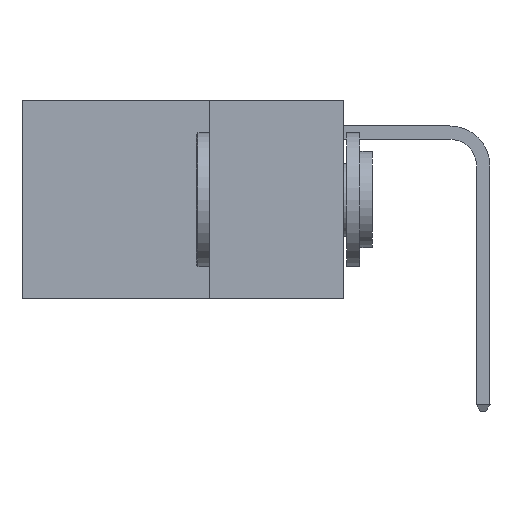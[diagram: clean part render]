
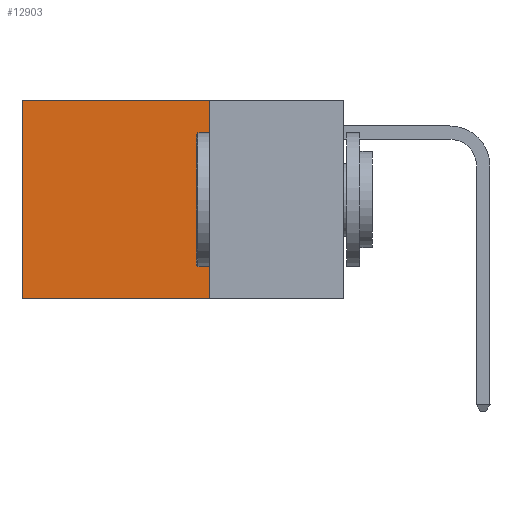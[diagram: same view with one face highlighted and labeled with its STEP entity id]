
A CAD part, left-side view. The second image highlights one B-rep face of the part: STEP entity #12903.
In plain terms, the highlighted planar face has unit normal (-1, 0, 0).
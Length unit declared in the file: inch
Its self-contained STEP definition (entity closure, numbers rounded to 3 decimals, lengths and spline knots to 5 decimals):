
#828 = CARTESIAN_POINT ( 'NONE',  ( 0.2625, 0.25, -0.37 ) ) ;
#1085 = VECTOR ( 'NONE', #15985, 39.37008 ) ;
#1234 = LINE ( 'NONE', #3697, #1085 ) ;
#2043 = ORIENTED_EDGE ( 'NONE', *, *, #5009, .T. ) ;
#2195 = ORIENTED_EDGE ( 'NONE', *, *, #12902, .F. ) ;
#2539 = EDGE_LOOP ( 'NONE', ( #5961, #2195, #7762, #2043 ) ) ;
#2912 = VECTOR ( 'NONE', #3433, 39.37008 ) ;
#3155 = DIRECTION ( 'NONE',  ( 0., 0., -1. ) ) ;
#3186 = DIRECTION ( 'NONE',  ( 1., 0., 0. ) ) ;
#3187 = CARTESIAN_POINT ( 'NONE',  ( 0.2625, 0.25, 0. ) ) ;
#3247 = PLANE ( 'NONE',  #5913 ) ;
#3404 = CARTESIAN_POINT ( 'NONE',  ( 0.2625, 0.25, -0.37 ) ) ;
#3433 = DIRECTION ( 'NONE',  ( 0., 1., 0. ) ) ;
#3697 = CARTESIAN_POINT ( 'NONE',  ( 0.2625, 0.6, 0. ) ) ;
#5009 = EDGE_CURVE ( 'NONE', #8512, #9461, #10351, .T. ) ;
#5743 = VERTEX_POINT ( 'NONE', #14196 ) ;
#5913 = AXIS2_PLACEMENT_3D ( 'NONE', #3187, #3186, #3155 ) ;
#5961 = ORIENTED_EDGE ( 'NONE', *, *, #7165, .T. ) ;
#6703 = DIRECTION ( 'NONE',  ( 0., 0., -1. ) ) ;
#7165 = EDGE_CURVE ( 'NONE', #9461, #5743, #1234, .T. ) ;
#7762 = ORIENTED_EDGE ( 'NONE', *, *, #14780, .F. ) ;
#7785 = LINE ( 'NONE', #15315, #13968 ) ;
#8512 = VERTEX_POINT ( 'NONE', #16199 ) ;
#8641 = CARTESIAN_POINT ( 'NONE',  ( 0.2625, 0.6, 0. ) ) ;
#9461 = VERTEX_POINT ( 'NONE', #8641 ) ;
#10306 = VECTOR ( 'NONE', #15509, 39.37008 ) ;
#10351 = LINE ( 'NONE', #15674, #10306 ) ;
#10502 = VERTEX_POINT ( 'NONE', #828 ) ;
#12674 = FACE_OUTER_BOUND ( 'NONE', #2539, .T. ) ;
#12902 = EDGE_CURVE ( 'NONE', #10502, #5743, #13079, .T. ) ;
#12903 = ADVANCED_FACE ( 'NONE', ( #12674 ), #3247, .F. ) ;
#13079 = LINE ( 'NONE', #3404, #2912 ) ;
#13968 = VECTOR ( 'NONE', #6703, 39.37008 ) ;
#14196 = CARTESIAN_POINT ( 'NONE',  ( 0.2625, 0.6, -0.37 ) ) ;
#14780 = EDGE_CURVE ( 'NONE', #8512, #10502, #7785, .T. ) ;
#15315 = CARTESIAN_POINT ( 'NONE',  ( 0.2625, 0.25, 0. ) ) ;
#15509 = DIRECTION ( 'NONE',  ( 0., 1., 0. ) ) ;
#15674 = CARTESIAN_POINT ( 'NONE',  ( 0.2625, 0.25, 0. ) ) ;
#15985 = DIRECTION ( 'NONE',  ( 0., 0., -1. ) ) ;
#16199 = CARTESIAN_POINT ( 'NONE',  ( 0.2625, 0.25, 0. ) ) ;
